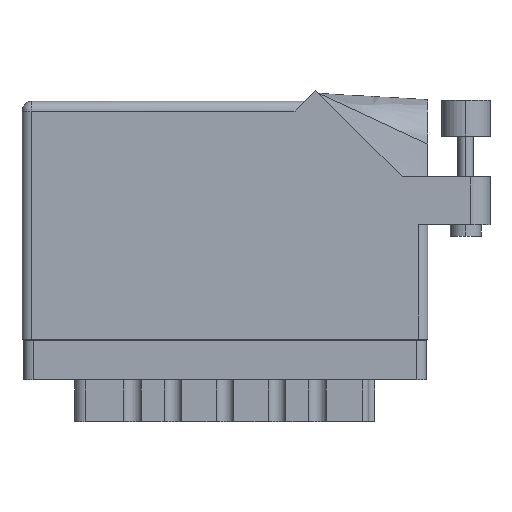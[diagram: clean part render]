
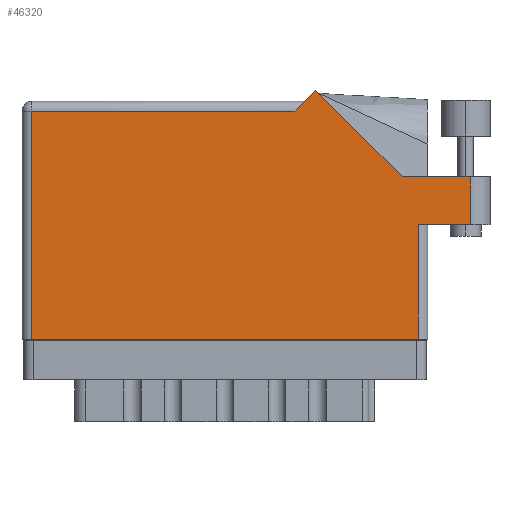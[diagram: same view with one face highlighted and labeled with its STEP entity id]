
A CAD part, front view. The second image highlights one B-rep face of the part: STEP entity #46320.
In plain terms, the highlighted face is planar.
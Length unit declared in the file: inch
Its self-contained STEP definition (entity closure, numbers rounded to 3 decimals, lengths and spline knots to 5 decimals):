
#1315 = VECTOR ( 'NONE', #18789, 39.37008 ) ;
#2059 = DIRECTION ( 'NONE',  ( -1., 0., 0. ) ) ;
#2371 = CARTESIAN_POINT ( 'NONE',  ( 2.887, 1.044, 0. ) ) ;
#3305 = VECTOR ( 'NONE', #33073, 39.37008 ) ;
#3511 = ORIENTED_EDGE ( 'NONE', *, *, #15406, .T. ) ;
#6993 = DIRECTION ( 'NONE',  ( -1., 0., 0. ) ) ;
#7213 = VERTEX_POINT ( 'NONE', #16093 ) ;
#7352 = PLANE ( 'NONE',  #44045 ) ;
#7656 = VECTOR ( 'NONE', #14499, 39.37008 ) ;
#8067 = CARTESIAN_POINT ( 'NONE',  ( 2.55, 0., 0. ) ) ;
#8113 = CARTESIAN_POINT ( 'NONE',  ( 2.887, 1.044, 0. ) ) ;
#9460 = VERTEX_POINT ( 'NONE', #8067 ) ;
#10586 = VERTEX_POINT ( 'NONE', #20035 ) ;
#10762 = DIRECTION ( 'NONE',  ( -1., 0., 0. ) ) ;
#10905 = VERTEX_POINT ( 'NONE', #11459 ) ;
#11459 = CARTESIAN_POINT ( 'NONE',  ( 1.88971, 1.60071, 0. ) ) ;
#11691 = VECTOR ( 'NONE', #10762, 39.37008 ) ;
#11895 = LINE ( 'NONE', #53348, #43007 ) ;
#12297 = VERTEX_POINT ( 'NONE', #21242 ) ;
#13431 = EDGE_CURVE ( 'NONE', #10905, #27425, #11895, .T. ) ;
#13609 = DIRECTION ( 'NONE',  ( 1., 0., 0. ) ) ;
#14499 = DIRECTION ( 'NONE',  ( -0.707, 0.707, 0. ) ) ;
#14506 = CARTESIAN_POINT ( 'NONE',  ( 3.012, 1.044, 0. ) ) ;
#14798 = DIRECTION ( 'NONE',  ( 0., -1., 0. ) ) ;
#15144 = CARTESIAN_POINT ( 'NONE',  ( 2.55, 0.737, 0. ) ) ;
#15406 = EDGE_CURVE ( 'NONE', #37438, #38019, #27260, .T. ) ;
#16093 = CARTESIAN_POINT ( 'NONE',  ( 0.062, 0., 0. ) ) ;
#17758 = EDGE_CURVE ( 'NONE', #38019, #10586, #36543, .T. ) ;
#18620 = CARTESIAN_POINT ( 'NONE',  ( 0.062, 0., 0. ) ) ;
#18789 = DIRECTION ( 'NONE',  ( 0., 1., 0. ) ) ;
#18822 = LINE ( 'NONE', #51313, #11691 ) ;
#19012 = EDGE_CURVE ( 'NONE', #34092, #37438, #24134, .T. ) ;
#19060 = CARTESIAN_POINT ( 'NONE',  ( 2.887, 0.737, 0. ) ) ;
#20035 = CARTESIAN_POINT ( 'NONE',  ( 2.44642, 1.044, 0. ) ) ;
#20839 = ORIENTED_EDGE ( 'NONE', *, *, #21877, .T. ) ;
#21105 = EDGE_CURVE ( 'NONE', #10586, #10905, #49070, .T. ) ;
#21242 = CARTESIAN_POINT ( 'NONE',  ( 0.062, 1.468, 0. ) ) ;
#21619 = CARTESIAN_POINT ( 'NONE',  ( 2.612, 0.737, 0. ) ) ;
#21877 = EDGE_CURVE ( 'NONE', #12297, #7213, #29633, .T. ) ;
#24134 = LINE ( 'NONE', #21619, #26070 ) ;
#24191 = DIRECTION ( 'NONE',  ( 1., 0., 0. ) ) ;
#24815 = ORIENTED_EDGE ( 'NONE', *, *, #27577, .T. ) ;
#25329 = EDGE_LOOP ( 'NONE', ( #26309, #3511, #45289, #53410, #40504, #41667, #20839, #24815, #43674 ) ) ;
#26070 = VECTOR ( 'NONE', #13609, 39.37008 ) ;
#26309 = ORIENTED_EDGE ( 'NONE', *, *, #19012, .T. ) ;
#27260 = LINE ( 'NONE', #8113, #3305 ) ;
#27425 = VERTEX_POINT ( 'NONE', #38660 ) ;
#27577 = EDGE_CURVE ( 'NONE', #7213, #9460, #44846, .T. ) ;
#28333 = VECTOR ( 'NONE', #14798, 39.37008 ) ;
#29125 = LINE ( 'NONE', #43567, #1315 ) ;
#29238 = EDGE_CURVE ( 'NONE', #9460, #34092, #29125, .T. ) ;
#29633 = LINE ( 'NONE', #18620, #28333 ) ;
#29959 = VECTOR ( 'NONE', #24191, 39.37008 ) ;
#33073 = DIRECTION ( 'NONE',  ( 0., 1., 0. ) ) ;
#33275 = DIRECTION ( 'NONE',  ( -0.707, -0.707, 0. ) ) ;
#34092 = VERTEX_POINT ( 'NONE', #15144 ) ;
#34579 = CARTESIAN_POINT ( 'NONE',  ( 2.44642, 1.044, 0. ) ) ;
#35868 = VECTOR ( 'NONE', #2059, 39.37008 ) ;
#36271 = CARTESIAN_POINT ( 'NONE',  ( 0., 1.53, 0. ) ) ;
#36543 = LINE ( 'NONE', #14506, #35868 ) ;
#37438 = VERTEX_POINT ( 'NONE', #19060 ) ;
#38019 = VERTEX_POINT ( 'NONE', #2371 ) ;
#38660 = CARTESIAN_POINT ( 'NONE',  ( 1.757, 1.468, 0. ) ) ;
#40504 = ORIENTED_EDGE ( 'NONE', *, *, #13431, .T. ) ;
#41667 = ORIENTED_EDGE ( 'NONE', *, *, #48920, .T. ) ;
#43007 = VECTOR ( 'NONE', #33275, 39.37008 ) ;
#43567 = CARTESIAN_POINT ( 'NONE',  ( 2.55, 0.737, 0. ) ) ;
#43674 = ORIENTED_EDGE ( 'NONE', *, *, #29238, .T. ) ;
#44045 = AXIS2_PLACEMENT_3D ( 'NONE', #36271, #52381, #6993 ) ;
#44846 = LINE ( 'NONE', #49105, #29959 ) ;
#45289 = ORIENTED_EDGE ( 'NONE', *, *, #17758, .T. ) ;
#45643 = FACE_OUTER_BOUND ( 'NONE', #25329, .T. ) ;
#46320 = ADVANCED_FACE ( 'NONE', ( #45643 ), #7352, .F. ) ;
#48920 = EDGE_CURVE ( 'NONE', #27425, #12297, #18822, .T. ) ;
#49070 = LINE ( 'NONE', #34579, #7656 ) ;
#49105 = CARTESIAN_POINT ( 'NONE',  ( 0., 0., 0. ) ) ;
#51313 = CARTESIAN_POINT ( 'NONE',  ( 0., 1.468, 0. ) ) ;
#52381 = DIRECTION ( 'NONE',  ( 0., 0., -1. ) ) ;
#53348 = CARTESIAN_POINT ( 'NONE',  ( 1.819, 1.53, 0. ) ) ;
#53410 = ORIENTED_EDGE ( 'NONE', *, *, #21105, .T. ) ;
